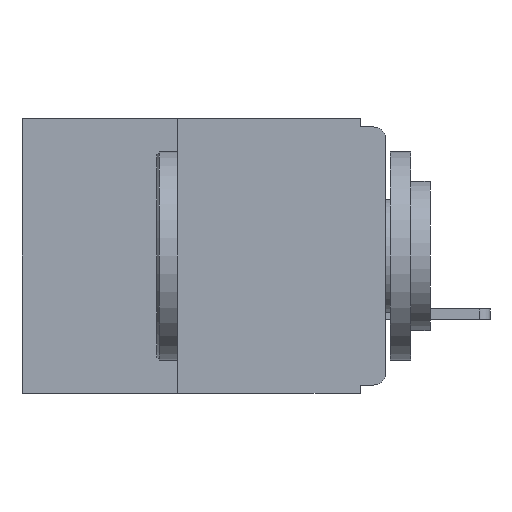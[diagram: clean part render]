
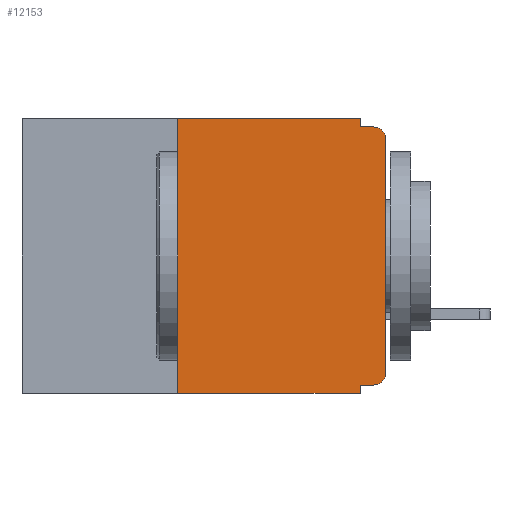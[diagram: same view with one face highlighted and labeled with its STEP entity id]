
A CAD part, left-side view. The second image highlights one B-rep face of the part: STEP entity #12153.
In plain terms, the highlighted planar face has unit normal (-1, 0, 0).
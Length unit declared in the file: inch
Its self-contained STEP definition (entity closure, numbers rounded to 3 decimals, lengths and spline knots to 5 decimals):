
#135 = PLANE ( 'NONE',  #6562 ) ;
#204 = DIRECTION ( 'NONE',  ( 0., 0., -1. ) ) ;
#324 = VERTEX_POINT ( 'NONE', #12176 ) ;
#1836 = DIRECTION ( 'NONE',  ( 0., 0., -1. ) ) ;
#1961 = CARTESIAN_POINT ( 'NONE',  ( 0., 0.031, -0.32 ) ) ;
#2036 = CARTESIAN_POINT ( 'NONE',  ( 0., 0.015, -0.025 ) ) ;
#2058 = LINE ( 'NONE', #12304, #5711 ) ;
#2099 = LINE ( 'NONE', #12709, #6304 ) ;
#2197 = CARTESIAN_POINT ( 'NONE',  ( 0., 0., -0.025 ) ) ;
#2702 = VERTEX_POINT ( 'NONE', #15701 ) ;
#2733 = VECTOR ( 'NONE', #14342, 39.37008 ) ;
#2763 = CARTESIAN_POINT ( 'NONE',  ( 0., 0.25, -0.33 ) ) ;
#2827 = ORIENTED_EDGE ( 'NONE', *, *, #11580, .T. ) ;
#3427 = CARTESIAN_POINT ( 'NONE',  ( 0., 0., -0.32 ) ) ;
#3665 = VERTEX_POINT ( 'NONE', #13404 ) ;
#3825 = DIRECTION ( 'NONE',  ( 0., 0., -1. ) ) ;
#3929 = CARTESIAN_POINT ( 'NONE',  ( 0., 0.031, -0.33 ) ) ;
#4405 = LINE ( 'NONE', #7472, #18183 ) ;
#4465 = CARTESIAN_POINT ( 'NONE',  ( 0., 0.015, -0.305 ) ) ;
#4558 = DIRECTION ( 'NONE',  ( 0., 0., 1. ) ) ;
#4807 = AXIS2_PLACEMENT_3D ( 'NONE', #4465, #16564, #6289 ) ;
#5711 = VECTOR ( 'NONE', #1836, 39.37008 ) ;
#6289 = DIRECTION ( 'NONE',  ( 0., 0., -1. ) ) ;
#6304 = VECTOR ( 'NONE', #16138, 39.37008 ) ;
#6562 = AXIS2_PLACEMENT_3D ( 'NONE', #20884, #10752, #204 ) ;
#7192 = VERTEX_POINT ( 'NONE', #15928 ) ;
#7472 = CARTESIAN_POINT ( 'NONE',  ( 0., 0.437, 0. ) ) ;
#7478 = VERTEX_POINT ( 'NONE', #13580 ) ;
#8194 = ORIENTED_EDGE ( 'NONE', *, *, #20628, .F. ) ;
#8233 = VERTEX_POINT ( 'NONE', #15667 ) ;
#8341 = FACE_OUTER_BOUND ( 'NONE', #9550, .T. ) ;
#8510 = CARTESIAN_POINT ( 'NONE',  ( 0., 0., 0. ) ) ;
#8853 = VECTOR ( 'NONE', #4558, 39.37008 ) ;
#9218 = CARTESIAN_POINT ( 'NONE',  ( 0., 0.437, -0.33 ) ) ;
#9439 = CARTESIAN_POINT ( 'NONE',  ( 0., 0.25, -0.33 ) ) ;
#9479 = ORIENTED_EDGE ( 'NONE', *, *, #15398, .T. ) ;
#9550 = EDGE_LOOP ( 'NONE', ( #14276, #19822, #12614, #22292, #14699, #8194, #2827, #11098, #19398, #9479 ) ) ;
#9773 = VECTOR ( 'NONE', #22068, 39.37008 ) ;
#9862 = EDGE_CURVE ( 'NONE', #3665, #12163, #21426, .T. ) ;
#9995 = EDGE_CURVE ( 'NONE', #21543, #324, #14274, .T. ) ;
#10752 = DIRECTION ( 'NONE',  ( 1., 0., 0. ) ) ;
#11066 = EDGE_CURVE ( 'NONE', #8233, #21543, #18265, .T. ) ;
#11098 = ORIENTED_EDGE ( 'NONE', *, *, #12878, .F. ) ;
#11580 = EDGE_CURVE ( 'NONE', #13412, #11601, #15566, .T. ) ;
#11601 = VERTEX_POINT ( 'NONE', #3929 ) ;
#12017 = LINE ( 'NONE', #12628, #2733 ) ;
#12153 = ADVANCED_FACE ( 'NONE', ( #8341 ), #135, .F. ) ;
#12163 = VERTEX_POINT ( 'NONE', #1961 ) ;
#12176 = CARTESIAN_POINT ( 'NONE',  ( 0., 0.015, -0.01 ) ) ;
#12304 = CARTESIAN_POINT ( 'NONE',  ( 0., 0.031, 0. ) ) ;
#12614 = ORIENTED_EDGE ( 'NONE', *, *, #14679, .F. ) ;
#12628 = CARTESIAN_POINT ( 'NONE',  ( 0., 0.031, -0.33 ) ) ;
#12709 = CARTESIAN_POINT ( 'NONE',  ( 0., 0., -0.01 ) ) ;
#12878 = EDGE_CURVE ( 'NONE', #12163, #11601, #12017, .T. ) ;
#13350 = LINE ( 'NONE', #2763, #8853 ) ;
#13404 = CARTESIAN_POINT ( 'NONE',  ( 0., 0.015, -0.32 ) ) ;
#13412 = VERTEX_POINT ( 'NONE', #9439 ) ;
#13580 = CARTESIAN_POINT ( 'NONE',  ( 0., 0.031, -0.01 ) ) ;
#14219 = DIRECTION ( 'NONE',  ( -1., 0., 0. ) ) ;
#14274 = CIRCLE ( 'NONE', #14577, 0.015 ) ;
#14276 = ORIENTED_EDGE ( 'NONE', *, *, #11066, .T. ) ;
#14342 = DIRECTION ( 'NONE',  ( 0., 0., -1. ) ) ;
#14577 = AXIS2_PLACEMENT_3D ( 'NONE', #2036, #14219, #3825 ) ;
#14679 = EDGE_CURVE ( 'NONE', #7478, #324, #2099, .T. ) ;
#14699 = ORIENTED_EDGE ( 'NONE', *, *, #20428, .F. ) ;
#15398 = EDGE_CURVE ( 'NONE', #3665, #8233, #18404, .T. ) ;
#15566 = LINE ( 'NONE', #9218, #16103 ) ;
#15667 = CARTESIAN_POINT ( 'NONE',  ( 0., 0., -0.305 ) ) ;
#15701 = CARTESIAN_POINT ( 'NONE',  ( 0., 0.25, 0. ) ) ;
#15928 = CARTESIAN_POINT ( 'NONE',  ( 0., 0.031, 0. ) ) ;
#16103 = VECTOR ( 'NONE', #21064, 39.37008 ) ;
#16138 = DIRECTION ( 'NONE',  ( 0., -1., 0. ) ) ;
#16564 = DIRECTION ( 'NONE',  ( -1., 0., 0. ) ) ;
#17084 = EDGE_CURVE ( 'NONE', #7192, #7478, #2058, .T. ) ;
#17303 = DIRECTION ( 'NONE',  ( 0., 1., 0. ) ) ;
#18183 = VECTOR ( 'NONE', #21067, 39.37008 ) ;
#18265 = LINE ( 'NONE', #8510, #9773 ) ;
#18404 = CIRCLE ( 'NONE', #4807, 0.015 ) ;
#19398 = ORIENTED_EDGE ( 'NONE', *, *, #9862, .F. ) ;
#19822 = ORIENTED_EDGE ( 'NONE', *, *, #9995, .T. ) ;
#20428 = EDGE_CURVE ( 'NONE', #2702, #7192, #4405, .T. ) ;
#20628 = EDGE_CURVE ( 'NONE', #13412, #2702, #13350, .T. ) ;
#20884 = CARTESIAN_POINT ( 'NONE',  ( 0., 0.437, 0. ) ) ;
#20899 = VECTOR ( 'NONE', #17303, 39.37008 ) ;
#21064 = DIRECTION ( 'NONE',  ( 0., -1., 0. ) ) ;
#21067 = DIRECTION ( 'NONE',  ( 0., -1., 0. ) ) ;
#21426 = LINE ( 'NONE', #3427, #20899 ) ;
#21543 = VERTEX_POINT ( 'NONE', #2197 ) ;
#22068 = DIRECTION ( 'NONE',  ( 0., 0., 1. ) ) ;
#22292 = ORIENTED_EDGE ( 'NONE', *, *, #17084, .F. ) ;
